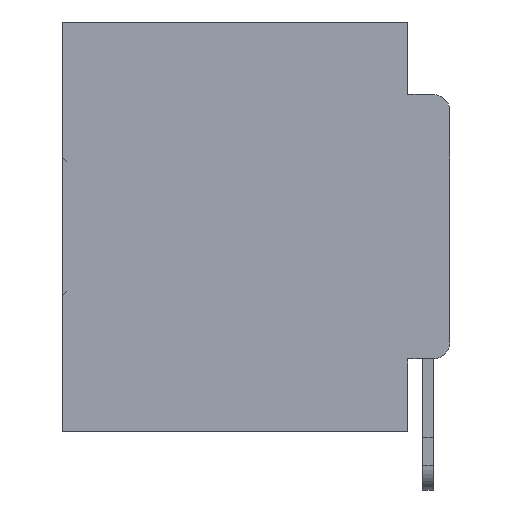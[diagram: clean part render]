
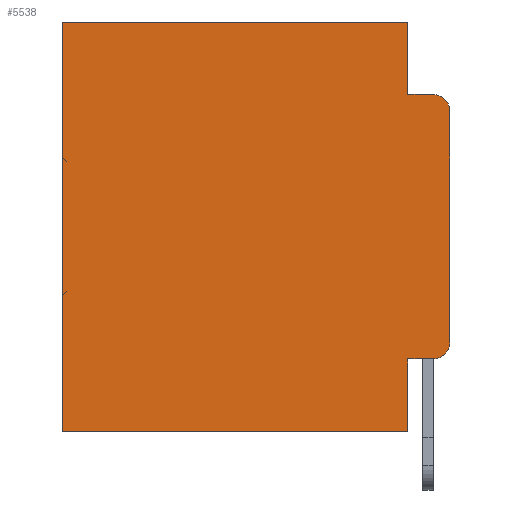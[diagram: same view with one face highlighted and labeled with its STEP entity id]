
A CAD part, left-side view. The second image highlights one B-rep face of the part: STEP entity #5538.
In plain terms, the highlighted planar face has unit normal (-1, 0, 0).
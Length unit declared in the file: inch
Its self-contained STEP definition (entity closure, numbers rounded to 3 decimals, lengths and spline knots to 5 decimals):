
#191 = VERTEX_POINT ( 'NONE', #20877 ) ;
#1021 = VERTEX_POINT ( 'NONE', #5739 ) ;
#1602 = LINE ( 'NONE', #23724, #14928 ) ;
#1762 = EDGE_CURVE ( 'NONE', #18056, #1021, #17402, .T. ) ;
#2095 = ORIENTED_EDGE ( 'NONE', *, *, #21231, .T. ) ;
#2415 = LINE ( 'NONE', #10255, #15720 ) ;
#2521 = ORIENTED_EDGE ( 'NONE', *, *, #10650, .F. ) ;
#2929 = CARTESIAN_POINT ( 'NONE',  ( 0.298, 0.473, 0. ) ) ;
#3100 = VECTOR ( 'NONE', #14132, 39.37008 ) ;
#3504 = CARTESIAN_POINT ( 'NONE',  ( 0.298, 0.02, -0.1085 ) ) ;
#3884 = ORIENTED_EDGE ( 'NONE', *, *, #6199, .F. ) ;
#4054 = VECTOR ( 'NONE', #32297, 39.37008 ) ;
#4149 = CARTESIAN_POINT ( 'NONE',  ( 0.298, 0.051, -0.4115 ) ) ;
#4510 = DIRECTION ( 'NONE',  ( 1., 0., 0. ) ) ;
#4633 = AXIS2_PLACEMENT_3D ( 'NONE', #20351, #4510, #22986 ) ;
#4672 = VECTOR ( 'NONE', #25283, 39.37008 ) ;
#5538 = ADVANCED_FACE ( 'NONE', ( #30136 ), #30915, .F. ) ;
#5558 = EDGE_LOOP ( 'NONE', ( #6475, #2095, #33954, #13916, #15913, #7258, #3884, #2521, #26128, #6576 ) ) ;
#5739 = CARTESIAN_POINT ( 'NONE',  ( 0.298, 0.473, -0.5 ) ) ;
#6170 = DIRECTION ( 'NONE',  ( 0., 0., -1. ) ) ;
#6199 = EDGE_CURVE ( 'NONE', #7723, #1021, #9881, .T. ) ;
#6310 = CARTESIAN_POINT ( 'NONE',  ( 0.298, 0., -0.3915 ) ) ;
#6426 = VERTEX_POINT ( 'NONE', #29314 ) ;
#6475 = ORIENTED_EDGE ( 'NONE', *, *, #7746, .F. ) ;
#6576 = ORIENTED_EDGE ( 'NONE', *, *, #23189, .T. ) ;
#7258 = ORIENTED_EDGE ( 'NONE', *, *, #1762, .T. ) ;
#7723 = VERTEX_POINT ( 'NONE', #21846 ) ;
#7746 = EDGE_CURVE ( 'NONE', #191, #19431, #28757, .T. ) ;
#8461 = CARTESIAN_POINT ( 'NONE',  ( 0.298, 0.051, 0. ) ) ;
#9078 = DIRECTION ( 'NONE',  ( 0., 0., -1. ) ) ;
#9188 = CARTESIAN_POINT ( 'NONE',  ( 0.298, 0.02, -0.3915 ) ) ;
#9541 = LINE ( 'NONE', #31349, #24388 ) ;
#9881 = LINE ( 'NONE', #20547, #29280 ) ;
#9889 = EDGE_CURVE ( 'NONE', #18532, #13951, #1602, .T. ) ;
#10255 = CARTESIAN_POINT ( 'NONE',  ( 0.298, 0.051, -0.0885 ) ) ;
#10352 = VERTEX_POINT ( 'NONE', #33694 ) ;
#10375 = VECTOR ( 'NONE', #9078, 39.37008 ) ;
#10650 = EDGE_CURVE ( 'NONE', #23272, #7723, #32233, .T. ) ;
#11470 = AXIS2_PLACEMENT_3D ( 'NONE', #3504, #22015, #6170 ) ;
#11870 = DIRECTION ( 'NONE',  ( 0., 0., -1. ) ) ;
#12850 = DIRECTION ( 'NONE',  ( 0., 1., 0. ) ) ;
#13916 = ORIENTED_EDGE ( 'NONE', *, *, #9889, .F. ) ;
#13951 = VERTEX_POINT ( 'NONE', #34179 ) ;
#14132 = DIRECTION ( 'NONE',  ( 0., 0., -1. ) ) ;
#14928 = VECTOR ( 'NONE', #21103, 39.37008 ) ;
#15158 = EDGE_CURVE ( 'NONE', #18532, #18056, #9541, .T. ) ;
#15720 = VECTOR ( 'NONE', #31539, 39.37008 ) ;
#15913 = ORIENTED_EDGE ( 'NONE', *, *, #15158, .T. ) ;
#16947 = CARTESIAN_POINT ( 'NONE',  ( 0.298, 0.473, 0. ) ) ;
#17367 = CIRCLE ( 'NONE', #25553, 0.02 ) ;
#17402 = LINE ( 'NONE', #16947, #10375 ) ;
#17888 = DIRECTION ( 'NONE',  ( 0., 1., 0. ) ) ;
#18056 = VERTEX_POINT ( 'NONE', #2929 ) ;
#18532 = VERTEX_POINT ( 'NONE', #20943 ) ;
#18960 = EDGE_CURVE ( 'NONE', #23272, #10352, #32842, .T. ) ;
#19431 = VERTEX_POINT ( 'NONE', #6310 ) ;
#20351 = CARTESIAN_POINT ( 'NONE',  ( 0.298, 0., 0. ) ) ;
#20547 = CARTESIAN_POINT ( 'NONE',  ( 0.298, 0., -0.5 ) ) ;
#20877 = CARTESIAN_POINT ( 'NONE',  ( 0.298, 0., -0.1085 ) ) ;
#20943 = CARTESIAN_POINT ( 'NONE',  ( 0.298, 0.051, 0. ) ) ;
#21103 = DIRECTION ( 'NONE',  ( 0., 0., -1. ) ) ;
#21231 = EDGE_CURVE ( 'NONE', #191, #6426, #28998, .T. ) ;
#21846 = CARTESIAN_POINT ( 'NONE',  ( 0.298, 0.051, -0.5 ) ) ;
#22015 = DIRECTION ( 'NONE',  ( -1., 0., 0. ) ) ;
#22681 = CARTESIAN_POINT ( 'NONE',  ( 0.298, 0.051, -0.4115 ) ) ;
#22986 = DIRECTION ( 'NONE',  ( 0., 0., -1. ) ) ;
#23189 = EDGE_CURVE ( 'NONE', #10352, #19431, #17367, .T. ) ;
#23272 = VERTEX_POINT ( 'NONE', #22681 ) ;
#23724 = CARTESIAN_POINT ( 'NONE',  ( 0.298, 0.051, 0. ) ) ;
#24388 = VECTOR ( 'NONE', #12850, 39.37008 ) ;
#25283 = DIRECTION ( 'NONE',  ( 0., -1., 0. ) ) ;
#25553 = AXIS2_PLACEMENT_3D ( 'NONE', #9188, #27657, #11870 ) ;
#26128 = ORIENTED_EDGE ( 'NONE', *, *, #18960, .T. ) ;
#27657 = DIRECTION ( 'NONE',  ( -1., 0., 0. ) ) ;
#28757 = LINE ( 'NONE', #29958, #3100 ) ;
#28998 = CIRCLE ( 'NONE', #11470, 0.02 ) ;
#29280 = VECTOR ( 'NONE', #17888, 39.37008 ) ;
#29314 = CARTESIAN_POINT ( 'NONE',  ( 0.298, 0.02, -0.0885 ) ) ;
#29958 = CARTESIAN_POINT ( 'NONE',  ( 0.298, 0., 0. ) ) ;
#30136 = FACE_OUTER_BOUND ( 'NONE', #5558, .T. ) ;
#30915 = PLANE ( 'NONE',  #4633 ) ;
#31349 = CARTESIAN_POINT ( 'NONE',  ( 0.298, 0., 0. ) ) ;
#31539 = DIRECTION ( 'NONE',  ( 0., -1., 0. ) ) ;
#32233 = LINE ( 'NONE', #8461, #4054 ) ;
#32297 = DIRECTION ( 'NONE',  ( 0., 0., -1. ) ) ;
#32842 = LINE ( 'NONE', #4149, #4672 ) ;
#33623 = EDGE_CURVE ( 'NONE', #13951, #6426, #2415, .T. ) ;
#33694 = CARTESIAN_POINT ( 'NONE',  ( 0.298, 0.02, -0.4115 ) ) ;
#33954 = ORIENTED_EDGE ( 'NONE', *, *, #33623, .F. ) ;
#34179 = CARTESIAN_POINT ( 'NONE',  ( 0.298, 0.051, -0.0885 ) ) ;
